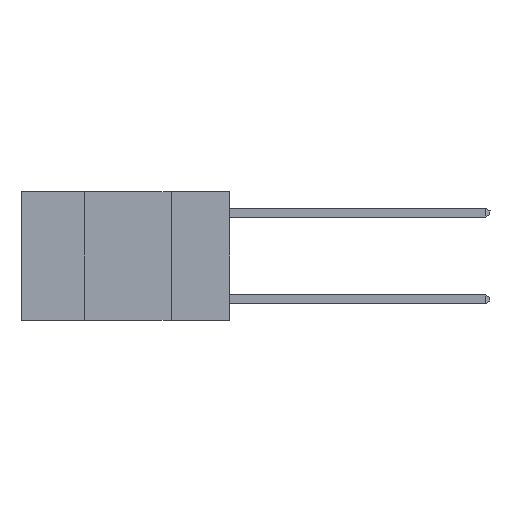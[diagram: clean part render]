
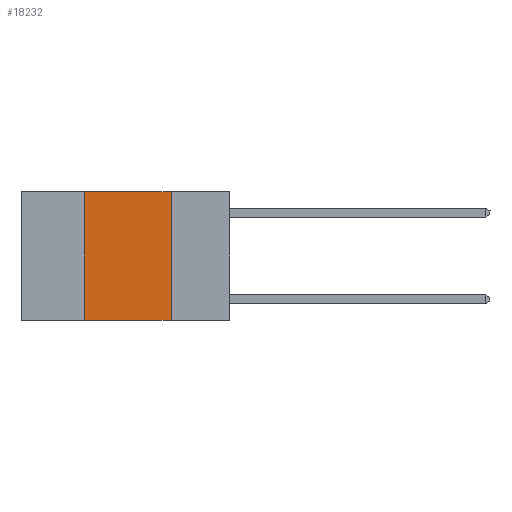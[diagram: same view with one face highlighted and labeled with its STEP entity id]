
A CAD part, left-side view. The second image highlights one B-rep face of the part: STEP entity #18232.
In plain terms, the highlighted planar face has unit normal (-1, 0, 0).
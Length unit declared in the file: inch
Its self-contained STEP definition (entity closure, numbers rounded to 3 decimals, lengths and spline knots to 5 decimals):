
#386 = DIRECTION ( 'NONE',  ( 0., -1., 0. ) ) ;
#897 = LINE ( 'NONE', #18368, #2942 ) ;
#1464 = EDGE_CURVE ( 'NONE', #10071, #2309, #897, .T. ) ;
#2214 = EDGE_CURVE ( 'NONE', #10071, #3269, #17948, .T. ) ;
#2309 = VERTEX_POINT ( 'NONE', #12798 ) ;
#2942 = VECTOR ( 'NONE', #3989, 39.37008 ) ;
#3269 = VERTEX_POINT ( 'NONE', #14590 ) ;
#3498 = CARTESIAN_POINT ( 'NONE',  ( 0., 0.17, 0. ) ) ;
#3989 = DIRECTION ( 'NONE',  ( 0., 0., 1. ) ) ;
#4951 = DIRECTION ( 'NONE',  ( 0., 0., -1. ) ) ;
#4952 = DIRECTION ( 'NONE',  ( 0., 0., -1. ) ) ;
#5038 = PLANE ( 'NONE',  #14129 ) ;
#5404 = CARTESIAN_POINT ( 'NONE',  ( 0., 0.6, 0. ) ) ;
#5596 = EDGE_CURVE ( 'NONE', #2309, #7624, #11357, .T. ) ;
#6795 = EDGE_CURVE ( 'NONE', #7624, #3269, #11085, .T. ) ;
#7624 = VERTEX_POINT ( 'NONE', #3498 ) ;
#8086 = ORIENTED_EDGE ( 'NONE', *, *, #6795, .F. ) ;
#9572 = CARTESIAN_POINT ( 'NONE',  ( 0., 0.6, 0. ) ) ;
#10071 = VERTEX_POINT ( 'NONE', #14314 ) ;
#11085 = LINE ( 'NONE', #18001, #16581 ) ;
#11357 = LINE ( 'NONE', #5404, #12506 ) ;
#12375 = ORIENTED_EDGE ( 'NONE', *, *, #2214, .T. ) ;
#12506 = VECTOR ( 'NONE', #15612, 39.37008 ) ;
#12798 = CARTESIAN_POINT ( 'NONE',  ( 0., 0.42, 0. ) ) ;
#12993 = ORIENTED_EDGE ( 'NONE', *, *, #5596, .F. ) ;
#13664 = FACE_OUTER_BOUND ( 'NONE', #16452, .T. ) ;
#14129 = AXIS2_PLACEMENT_3D ( 'NONE', #9572, #18192, #4952 ) ;
#14314 = CARTESIAN_POINT ( 'NONE',  ( 0., 0.42, -0.37 ) ) ;
#14590 = CARTESIAN_POINT ( 'NONE',  ( 0., 0.17, -0.37 ) ) ;
#15612 = DIRECTION ( 'NONE',  ( 0., -1., 0. ) ) ;
#16341 = CARTESIAN_POINT ( 'NONE',  ( 0., 0.6, -0.37 ) ) ;
#16452 = EDGE_LOOP ( 'NONE', ( #8086, #12993, #17796, #12375 ) ) ;
#16581 = VECTOR ( 'NONE', #4951, 39.37008 ) ;
#17796 = ORIENTED_EDGE ( 'NONE', *, *, #1464, .F. ) ;
#17948 = LINE ( 'NONE', #16341, #18661 ) ;
#18001 = CARTESIAN_POINT ( 'NONE',  ( 0., 0.17, 0. ) ) ;
#18192 = DIRECTION ( 'NONE',  ( 1., 0., 0. ) ) ;
#18232 = ADVANCED_FACE ( 'NONE', ( #13664 ), #5038, .F. ) ;
#18368 = CARTESIAN_POINT ( 'NONE',  ( 0., 0.42, 0. ) ) ;
#18661 = VECTOR ( 'NONE', #386, 39.37008 ) ;
